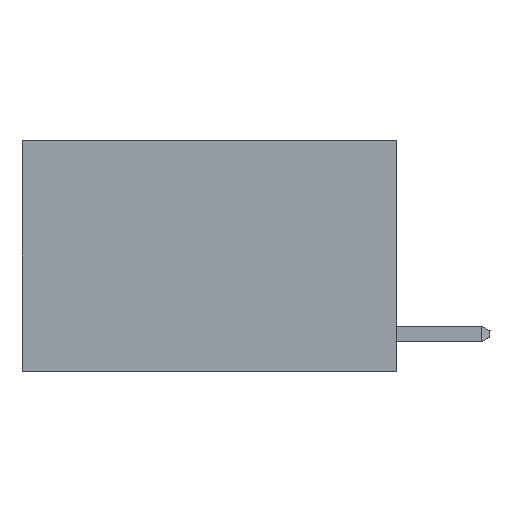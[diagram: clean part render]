
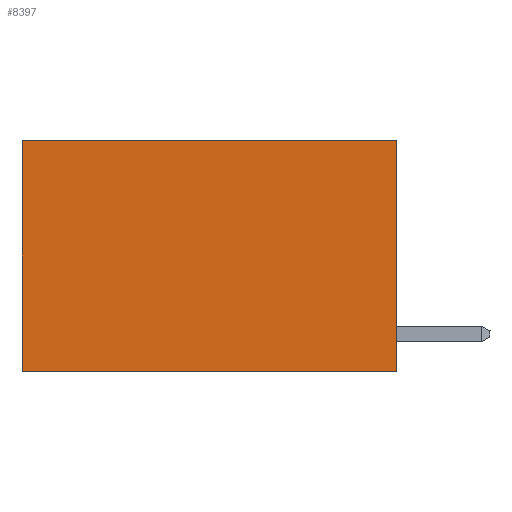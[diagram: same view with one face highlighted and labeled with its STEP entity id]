
A CAD part, left-side view. The second image highlights one B-rep face of the part: STEP entity #8397.
In plain terms, the highlighted planar face has unit normal (-1, 0, 0).
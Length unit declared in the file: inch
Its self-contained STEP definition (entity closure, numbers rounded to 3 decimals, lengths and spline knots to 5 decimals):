
#691 = AXIS2_PLACEMENT_3D ( 'NONE', #13340, #8115, #14572 ) ;
#1055 = CARTESIAN_POINT ( 'NONE',  ( 0.2625, 0., 0. ) ) ;
#1756 = CARTESIAN_POINT ( 'NONE',  ( 0.2625, 0., 0. ) ) ;
#1938 = CARTESIAN_POINT ( 'NONE',  ( 0.2625, 0.6, 0. ) ) ;
#1950 = ORIENTED_EDGE ( 'NONE', *, *, #3552, .T. ) ;
#2012 = EDGE_CURVE ( 'NONE', #10411, #11842, #6252, .T. ) ;
#2093 = LINE ( 'NONE', #1938, #13515 ) ;
#2434 = DIRECTION ( 'NONE',  ( 0., 0., -1. ) ) ;
#3552 = EDGE_CURVE ( 'NONE', #10411, #6328, #15314, .T. ) ;
#4897 = DIRECTION ( 'NONE',  ( 0., 0., -1. ) ) ;
#5093 = VECTOR ( 'NONE', #12148, 39.37008 ) ;
#5243 = VECTOR ( 'NONE', #2434, 39.37008 ) ;
#6252 = LINE ( 'NONE', #1055, #5243 ) ;
#6328 = VERTEX_POINT ( 'NONE', #11004 ) ;
#6832 = CARTESIAN_POINT ( 'NONE',  ( 0.2625, 0., 0. ) ) ;
#7132 = PLANE ( 'NONE',  #691 ) ;
#7167 = CARTESIAN_POINT ( 'NONE',  ( 0.2625, 0., -0.37 ) ) ;
#7503 = CARTESIAN_POINT ( 'NONE',  ( 0.2625, 0., -0.37 ) ) ;
#8047 = DIRECTION ( 'NONE',  ( 0., 1., 0. ) ) ;
#8115 = DIRECTION ( 'NONE',  ( 1., 0., 0. ) ) ;
#8397 = ADVANCED_FACE ( 'NONE', ( #11713 ), #7132, .F. ) ;
#9811 = ORIENTED_EDGE ( 'NONE', *, *, #12289, .F. ) ;
#10014 = EDGE_LOOP ( 'NONE', ( #13383, #9811, #10039, #1950 ) ) ;
#10039 = ORIENTED_EDGE ( 'NONE', *, *, #2012, .F. ) ;
#10411 = VERTEX_POINT ( 'NONE', #1756 ) ;
#10658 = VECTOR ( 'NONE', #8047, 39.37008 ) ;
#11004 = CARTESIAN_POINT ( 'NONE',  ( 0.2625, 0.6, 0. ) ) ;
#11713 = FACE_OUTER_BOUND ( 'NONE', #10014, .T. ) ;
#11842 = VERTEX_POINT ( 'NONE', #7503 ) ;
#12148 = DIRECTION ( 'NONE',  ( 0., 1., 0. ) ) ;
#12289 = EDGE_CURVE ( 'NONE', #11842, #15838, #13373, .T. ) ;
#12960 = CARTESIAN_POINT ( 'NONE',  ( 0.2625, 0.6, -0.37 ) ) ;
#13340 = CARTESIAN_POINT ( 'NONE',  ( 0.2625, 0., 0. ) ) ;
#13373 = LINE ( 'NONE', #7167, #5093 ) ;
#13383 = ORIENTED_EDGE ( 'NONE', *, *, #15125, .T. ) ;
#13515 = VECTOR ( 'NONE', #4897, 39.37008 ) ;
#14572 = DIRECTION ( 'NONE',  ( 0., 0., -1. ) ) ;
#15125 = EDGE_CURVE ( 'NONE', #6328, #15838, #2093, .T. ) ;
#15314 = LINE ( 'NONE', #6832, #10658 ) ;
#15838 = VERTEX_POINT ( 'NONE', #12960 ) ;
